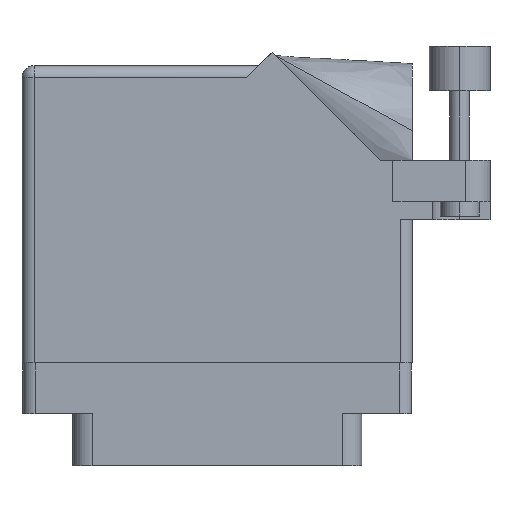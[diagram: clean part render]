
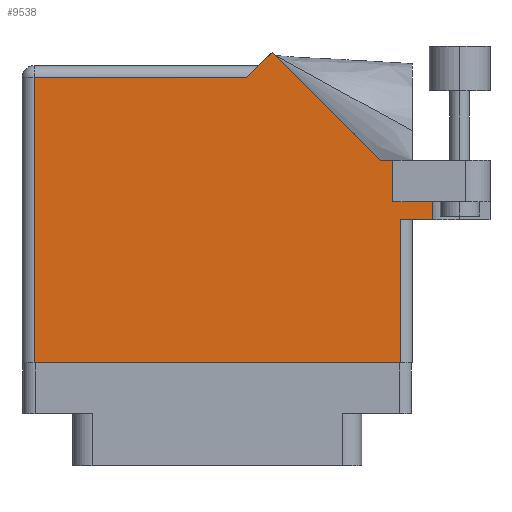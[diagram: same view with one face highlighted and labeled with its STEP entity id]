
A CAD part, front view. The second image highlights one B-rep face of the part: STEP entity #9538.
In plain terms, the highlighted face is planar.
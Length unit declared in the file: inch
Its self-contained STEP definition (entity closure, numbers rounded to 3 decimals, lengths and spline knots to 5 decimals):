
#269 = VECTOR ( 'NONE', #10637, 39.37008 ) ;
#327 = VERTEX_POINT ( 'NONE', #16219 ) ;
#540 = DIRECTION ( 'NONE',  ( -0.707, 0.707, 0. ) ) ;
#793 = ORIENTED_EDGE ( 'NONE', *, *, #18934, .T. ) ;
#851 = CARTESIAN_POINT ( 'NONE',  ( 0., 1.53, 0. ) ) ;
#892 = CARTESIAN_POINT ( 'NONE',  ( 1.84442, 1.044, 0. ) ) ;
#1534 = VECTOR ( 'NONE', #15969, 39.37008 ) ;
#1756 = VECTOR ( 'NONE', #8941, 39.37008 ) ;
#1812 = VERTEX_POINT ( 'NONE', #10441 ) ;
#2496 = CARTESIAN_POINT ( 'NONE',  ( 2.01, 0.737, 0. ) ) ;
#2752 = LINE ( 'NONE', #11264, #24098 ) ;
#2873 = DIRECTION ( 'NONE',  ( 0., -1., 0. ) ) ;
#2916 = DIRECTION ( 'NONE',  ( -0.707, -0.707, 0. ) ) ;
#2939 = LINE ( 'NONE', #892, #28211 ) ;
#3585 = DIRECTION ( 'NONE',  ( -1., 0., 0. ) ) ;
#3816 = PLANE ( 'NONE',  #25254 ) ;
#3886 = LINE ( 'NONE', #20366, #24399 ) ;
#4097 = LINE ( 'NONE', #27115, #269 ) ;
#4429 = CARTESIAN_POINT ( 'NONE',  ( 1.84442, 1.044, 0. ) ) ;
#6353 = DIRECTION ( 'NONE',  ( 0., 0., -1. ) ) ;
#6801 = CARTESIAN_POINT ( 'NONE',  ( 2.1115, 0.831, 0. ) ) ;
#6863 = VERTEX_POINT ( 'NONE', #13723 ) ;
#7088 = EDGE_CURVE ( 'NONE', #30186, #22060, #14883, .T. ) ;
#7494 = VECTOR ( 'NONE', #21615, 39.37008 ) ;
#7625 = EDGE_CURVE ( 'NONE', #1812, #30186, #17363, .T. ) ;
#7930 = FACE_OUTER_BOUND ( 'NONE', #24021, .T. ) ;
#8261 = CARTESIAN_POINT ( 'NONE',  ( 2.1115, 0.737, 0. ) ) ;
#8941 = DIRECTION ( 'NONE',  ( 1., 0., 0. ) ) ;
#9538 = ADVANCED_FACE ( 'NONE', ( #7930 ), #3816, .F. ) ;
#9770 = VECTOR ( 'NONE', #12272, 39.37008 ) ;
#10000 = ORIENTED_EDGE ( 'NONE', *, *, #7088, .T. ) ;
#10441 = CARTESIAN_POINT ( 'NONE',  ( 1.28771, 1.60071, 0. ) ) ;
#10637 = DIRECTION ( 'NONE',  ( 0., 1., 0. ) ) ;
#11264 = CARTESIAN_POINT ( 'NONE',  ( 2.1115, 1.16177, 0. ) ) ;
#12218 = VERTEX_POINT ( 'NONE', #6801 ) ;
#12272 = DIRECTION ( 'NONE',  ( -1., 0., 0. ) ) ;
#12610 = DIRECTION ( 'NONE',  ( 1., 0., 0. ) ) ;
#12789 = ORIENTED_EDGE ( 'NONE', *, *, #29152, .F. ) ;
#12846 = EDGE_CURVE ( 'NONE', #27103, #1812, #2939, .T. ) ;
#13148 = VERTEX_POINT ( 'NONE', #35347 ) ;
#13333 = EDGE_CURVE ( 'NONE', #12218, #14578, #2752, .T. ) ;
#13368 = ORIENTED_EDGE ( 'NONE', *, *, #27211, .T. ) ;
#13723 = CARTESIAN_POINT ( 'NONE',  ( 1.91, 1.044, 0. ) ) ;
#14578 = VERTEX_POINT ( 'NONE', #8261 ) ;
#14883 = LINE ( 'NONE', #28894, #9770 ) ;
#15411 = ORIENTED_EDGE ( 'NONE', *, *, #33034, .T. ) ;
#15969 = DIRECTION ( 'NONE',  ( 0., 1., 0. ) ) ;
#16219 = CARTESIAN_POINT ( 'NONE',  ( 1.91, 0.831, 0. ) ) ;
#17185 = ORIENTED_EDGE ( 'NONE', *, *, #22054, .T. ) ;
#17363 = LINE ( 'NONE', #22278, #28514 ) ;
#17582 = CARTESIAN_POINT ( 'NONE',  ( 0.062, 1.468, 0. ) ) ;
#17689 = LINE ( 'NONE', #2496, #7494 ) ;
#18235 = LINE ( 'NONE', #31015, #28109 ) ;
#18408 = VERTEX_POINT ( 'NONE', #22788 ) ;
#18934 = EDGE_CURVE ( 'NONE', #6863, #27103, #20363, .T. ) ;
#20139 = CARTESIAN_POINT ( 'NONE',  ( 2.41, 1.044, 0. ) ) ;
#20213 = DIRECTION ( 'NONE',  ( 0., -1., 0. ) ) ;
#20363 = LINE ( 'NONE', #20139, #26798 ) ;
#20366 = CARTESIAN_POINT ( 'NONE',  ( 0., 0., 0. ) ) ;
#21615 = DIRECTION ( 'NONE',  ( 1., 0., 0. ) ) ;
#22054 = EDGE_CURVE ( 'NONE', #22060, #18408, #18235, .T. ) ;
#22060 = VERTEX_POINT ( 'NONE', #17582 ) ;
#22278 = CARTESIAN_POINT ( 'NONE',  ( 1.217, 1.53, 0. ) ) ;
#22516 = DIRECTION ( 'NONE',  ( -1., 0., 0. ) ) ;
#22788 = CARTESIAN_POINT ( 'NONE',  ( 0.062, 0., 0. ) ) ;
#22833 = ORIENTED_EDGE ( 'NONE', *, *, #26327, .T. ) ;
#24021 = EDGE_LOOP ( 'NONE', ( #22833, #15411, #13368, #33467, #12789, #30119, #793, #31689, #32702, #10000, #17185 ) ) ;
#24098 = VECTOR ( 'NONE', #2873, 39.37008 ) ;
#24399 = VECTOR ( 'NONE', #12610, 39.37008 ) ;
#25254 = AXIS2_PLACEMENT_3D ( 'NONE', #851, #6353, #3585 ) ;
#26327 = EDGE_CURVE ( 'NONE', #18408, #13148, #3886, .T. ) ;
#26798 = VECTOR ( 'NONE', #22516, 39.37008 ) ;
#27103 = VERTEX_POINT ( 'NONE', #4429 ) ;
#27115 = CARTESIAN_POINT ( 'NONE',  ( 1.948, 0.737, 0. ) ) ;
#27211 = EDGE_CURVE ( 'NONE', #32058, #14578, #17689, .T. ) ;
#28109 = VECTOR ( 'NONE', #20213, 39.37008 ) ;
#28211 = VECTOR ( 'NONE', #540, 39.37008 ) ;
#28432 = CARTESIAN_POINT ( 'NONE',  ( 1.155, 1.468, 0. ) ) ;
#28514 = VECTOR ( 'NONE', #2916, 39.37008 ) ;
#28894 = CARTESIAN_POINT ( 'NONE',  ( 0., 1.468, 0. ) ) ;
#28914 = LINE ( 'NONE', #34730, #1534 ) ;
#29152 = EDGE_CURVE ( 'NONE', #327, #12218, #33477, .T. ) ;
#30119 = ORIENTED_EDGE ( 'NONE', *, *, #32928, .T. ) ;
#30186 = VERTEX_POINT ( 'NONE', #28432 ) ;
#30812 = CARTESIAN_POINT ( 'NONE',  ( 1.91, 0.831, 0. ) ) ;
#31015 = CARTESIAN_POINT ( 'NONE',  ( 0.062, 0., 0. ) ) ;
#31689 = ORIENTED_EDGE ( 'NONE', *, *, #12846, .T. ) ;
#32058 = VERTEX_POINT ( 'NONE', #32852 ) ;
#32702 = ORIENTED_EDGE ( 'NONE', *, *, #7625, .T. ) ;
#32852 = CARTESIAN_POINT ( 'NONE',  ( 1.948, 0.737, 0. ) ) ;
#32928 = EDGE_CURVE ( 'NONE', #327, #6863, #28914, .T. ) ;
#33034 = EDGE_CURVE ( 'NONE', #13148, #32058, #4097, .T. ) ;
#33467 = ORIENTED_EDGE ( 'NONE', *, *, #13333, .F. ) ;
#33477 = LINE ( 'NONE', #30812, #1756 ) ;
#34730 = CARTESIAN_POINT ( 'NONE',  ( 1.91, 0.831, 0. ) ) ;
#35347 = CARTESIAN_POINT ( 'NONE',  ( 1.948, 0., 0. ) ) ;
